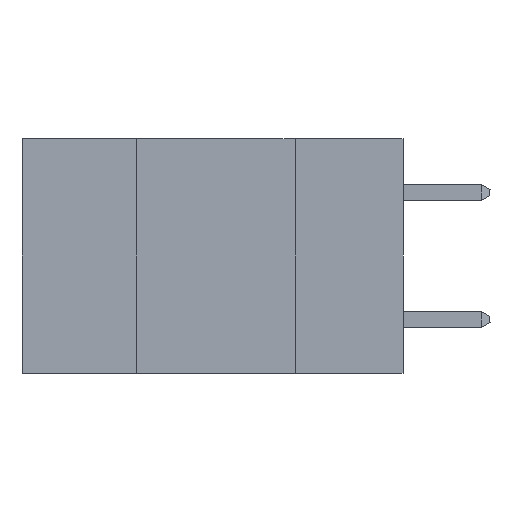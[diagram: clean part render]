
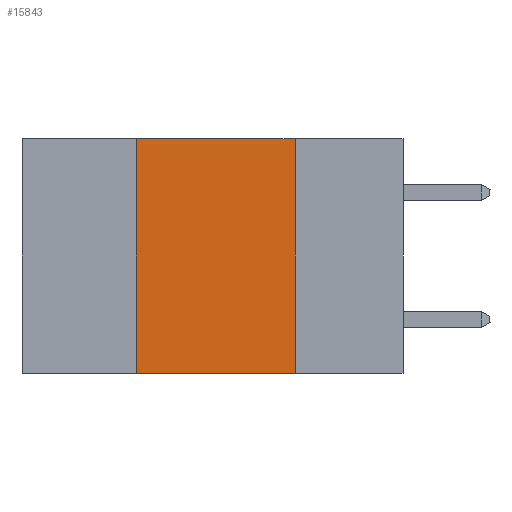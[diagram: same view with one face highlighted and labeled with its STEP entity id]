
A CAD part, left-side view. The second image highlights one B-rep face of the part: STEP entity #15843.
In plain terms, the highlighted planar face has unit normal (-1, 0, 0).
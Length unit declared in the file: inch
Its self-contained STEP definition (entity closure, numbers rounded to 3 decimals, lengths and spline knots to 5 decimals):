
#737 = DIRECTION ( 'NONE',  ( 0., -1., 0. ) ) ;
#1493 = EDGE_CURVE ( 'NONE', #6017, #15258, #9863, .T. ) ;
#1518 = CARTESIAN_POINT ( 'NONE',  ( 0., 0.17, -0.37 ) ) ;
#2233 = ORIENTED_EDGE ( 'NONE', *, *, #16812, .F. ) ;
#2635 = VERTEX_POINT ( 'NONE', #20487 ) ;
#2869 = CARTESIAN_POINT ( 'NONE',  ( 0., 0.42, 0. ) ) ;
#3557 = EDGE_CURVE ( 'NONE', #2635, #15258, #8980, .T. ) ;
#3733 = VERTEX_POINT ( 'NONE', #2869 ) ;
#4180 = CARTESIAN_POINT ( 'NONE',  ( 0., 0.6, 0. ) ) ;
#4454 = VECTOR ( 'NONE', #737, 39.37008 ) ;
#4691 = EDGE_LOOP ( 'NONE', ( #19183, #6221, #2233, #7304 ) ) ;
#5417 = DIRECTION ( 'NONE',  ( 0., 0., 1. ) ) ;
#5470 = AXIS2_PLACEMENT_3D ( 'NONE', #16627, #6500, #18317 ) ;
#5491 = CARTESIAN_POINT ( 'NONE',  ( 0., 0.42, 0. ) ) ;
#5519 = LINE ( 'NONE', #4180, #18491 ) ;
#5883 = DIRECTION ( 'NONE',  ( 0., -1., 0. ) ) ;
#6017 = VERTEX_POINT ( 'NONE', #13088 ) ;
#6221 = ORIENTED_EDGE ( 'NONE', *, *, #17183, .F. ) ;
#6500 = DIRECTION ( 'NONE',  ( 1., 0., 0. ) ) ;
#7304 = ORIENTED_EDGE ( 'NONE', *, *, #3557, .T. ) ;
#7943 = VECTOR ( 'NONE', #5417, 39.37008 ) ;
#8980 = LINE ( 'NONE', #9193, #4454 ) ;
#9193 = CARTESIAN_POINT ( 'NONE',  ( 0., 0.6, -0.37 ) ) ;
#9863 = LINE ( 'NONE', #13932, #21706 ) ;
#13088 = CARTESIAN_POINT ( 'NONE',  ( 0., 0.17, 0. ) ) ;
#13510 = LINE ( 'NONE', #5491, #7943 ) ;
#13913 = DIRECTION ( 'NONE',  ( 0., 0., -1. ) ) ;
#13932 = CARTESIAN_POINT ( 'NONE',  ( 0., 0.17, 0. ) ) ;
#14073 = FACE_OUTER_BOUND ( 'NONE', #4691, .T. ) ;
#15258 = VERTEX_POINT ( 'NONE', #1518 ) ;
#15843 = ADVANCED_FACE ( 'NONE', ( #14073 ), #19937, .F. ) ;
#16627 = CARTESIAN_POINT ( 'NONE',  ( 0., 0.6, 0. ) ) ;
#16812 = EDGE_CURVE ( 'NONE', #2635, #3733, #13510, .T. ) ;
#17183 = EDGE_CURVE ( 'NONE', #3733, #6017, #5519, .T. ) ;
#18317 = DIRECTION ( 'NONE',  ( 0., 0., -1. ) ) ;
#18491 = VECTOR ( 'NONE', #5883, 39.37008 ) ;
#19183 = ORIENTED_EDGE ( 'NONE', *, *, #1493, .F. ) ;
#19937 = PLANE ( 'NONE',  #5470 ) ;
#20487 = CARTESIAN_POINT ( 'NONE',  ( 0., 0.42, -0.37 ) ) ;
#21706 = VECTOR ( 'NONE', #13913, 39.37008 ) ;
